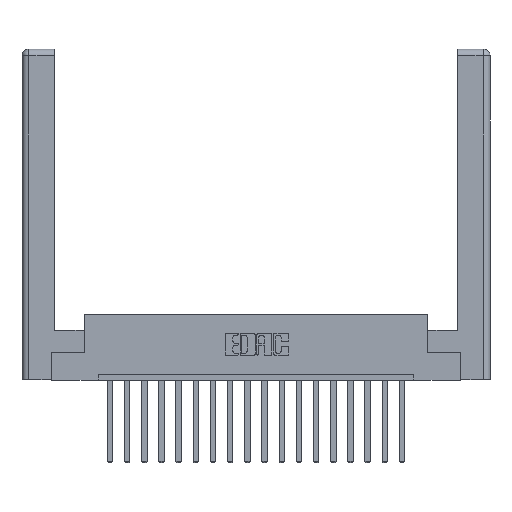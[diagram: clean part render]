
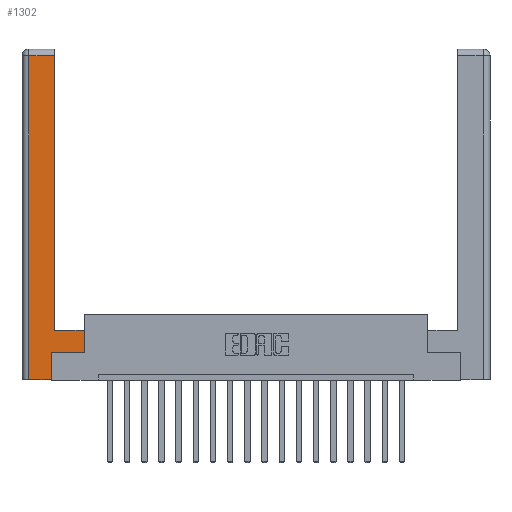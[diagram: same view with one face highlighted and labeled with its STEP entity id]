
A CAD part, top view. The second image highlights one B-rep face of the part: STEP entity #1302.
In plain terms, the highlighted planar face has unit normal (0, 0, 1).
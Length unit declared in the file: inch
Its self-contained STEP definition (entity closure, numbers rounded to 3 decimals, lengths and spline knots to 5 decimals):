
#709 = ORIENTED_EDGE ( 'NONE', *, *, #9413, .T. ) ;
#1058 = VECTOR ( 'NONE', #8706, 39.37008 ) ;
#1302 = ADVANCED_FACE ( 'NONE', ( #15863 ), #8562, .F. ) ;
#1546 = CARTESIAN_POINT ( 'NONE',  ( 0.565, 0.245, 0. ) ) ;
#1646 = VERTEX_POINT ( 'NONE', #6584 ) ;
#2027 = EDGE_CURVE ( 'NONE', #1646, #18087, #2345, .T. ) ;
#2048 = CARTESIAN_POINT ( 'NONE',  ( 0.265, 0., 0. ) ) ;
#2218 = EDGE_CURVE ( 'NONE', #15496, #9915, #7611, .T. ) ;
#2339 = DIRECTION ( 'NONE',  ( 0., 1., 0. ) ) ;
#2345 = LINE ( 'NONE', #8166, #11523 ) ;
#2350 = LINE ( 'NONE', #13489, #13578 ) ;
#2650 = CARTESIAN_POINT ( 'NONE',  ( 0.0615, 2.94, 0. ) ) ;
#2693 = CARTESIAN_POINT ( 'NONE',  ( 0.265, 0., 0. ) ) ;
#2729 = DIRECTION ( 'NONE',  ( -1., 0., 0. ) ) ;
#3001 = DIRECTION ( 'NONE',  ( 1., 0., 0. ) ) ;
#3193 = VECTOR ( 'NONE', #13538, 39.37008 ) ;
#3592 = EDGE_CURVE ( 'NONE', #9915, #18809, #2350, .T. ) ;
#4389 = CARTESIAN_POINT ( 'NONE',  ( 0.0615, 0., 0. ) ) ;
#4455 = ORIENTED_EDGE ( 'NONE', *, *, #3592, .T. ) ;
#4514 = DIRECTION ( 'NONE',  ( 0., 1., 0. ) ) ;
#4628 = VERTEX_POINT ( 'NONE', #2693 ) ;
#4725 = ORIENTED_EDGE ( 'NONE', *, *, #18942, .T. ) ;
#5455 = CARTESIAN_POINT ( 'NONE',  ( 0.0615, 0., 0. ) ) ;
#6584 = CARTESIAN_POINT ( 'NONE',  ( 0.295, 0.45, 0. ) ) ;
#7130 = CARTESIAN_POINT ( 'NONE',  ( 0., 0., 0. ) ) ;
#7320 = LINE ( 'NONE', #2048, #8725 ) ;
#7611 = LINE ( 'NONE', #1546, #9930 ) ;
#8067 = CARTESIAN_POINT ( 'NONE',  ( 0.0615, 2.94, 0. ) ) ;
#8166 = CARTESIAN_POINT ( 'NONE',  ( 0.295, 3., 0. ) ) ;
#8175 = VECTOR ( 'NONE', #17432, 39.37008 ) ;
#8516 = VERTEX_POINT ( 'NONE', #8067 ) ;
#8562 = PLANE ( 'NONE',  #10158 ) ;
#8706 = DIRECTION ( 'NONE',  ( 0., -1., 0. ) ) ;
#8714 = LINE ( 'NONE', #2650, #9632 ) ;
#8725 = VECTOR ( 'NONE', #14958, 39.37008 ) ;
#9068 = CARTESIAN_POINT ( 'NONE',  ( 0.265, 0.245, 0. ) ) ;
#9328 = LINE ( 'NONE', #4389, #1058 ) ;
#9413 = EDGE_CURVE ( 'NONE', #4628, #15496, #12985, .T. ) ;
#9632 = VECTOR ( 'NONE', #14292, 39.37008 ) ;
#9915 = VERTEX_POINT ( 'NONE', #14558 ) ;
#9930 = VECTOR ( 'NONE', #3001, 39.37008 ) ;
#10158 = AXIS2_PLACEMENT_3D ( 'NONE', #7130, #14496, #2729 ) ;
#10539 = CARTESIAN_POINT ( 'NONE',  ( 0.295, 0.45, 0. ) ) ;
#10904 = ORIENTED_EDGE ( 'NONE', *, *, #2218, .T. ) ;
#11028 = ORIENTED_EDGE ( 'NONE', *, *, #12440, .T. ) ;
#11227 = CARTESIAN_POINT ( 'NONE',  ( 0.295, 2.94, 0. ) ) ;
#11523 = VECTOR ( 'NONE', #2339, 39.37008 ) ;
#12440 = EDGE_CURVE ( 'NONE', #18087, #8516, #8714, .T. ) ;
#12825 = LINE ( 'NONE', #10539, #3193 ) ;
#12985 = LINE ( 'NONE', #18950, #8175 ) ;
#13014 = ORIENTED_EDGE ( 'NONE', *, *, #2027, .T. ) ;
#13489 = CARTESIAN_POINT ( 'NONE',  ( 0.565, 0.45, 0. ) ) ;
#13538 = DIRECTION ( 'NONE',  ( -1., 0., 0. ) ) ;
#13578 = VECTOR ( 'NONE', #4514, 39.37008 ) ;
#13657 = VERTEX_POINT ( 'NONE', #5455 ) ;
#13859 = ORIENTED_EDGE ( 'NONE', *, *, #17811, .T. ) ;
#14292 = DIRECTION ( 'NONE',  ( -1., 0., 0. ) ) ;
#14496 = DIRECTION ( 'NONE',  ( 0., 0., -1. ) ) ;
#14558 = CARTESIAN_POINT ( 'NONE',  ( 0.565, 0.245, 0. ) ) ;
#14958 = DIRECTION ( 'NONE',  ( 1., 0., 0. ) ) ;
#14987 = EDGE_CURVE ( 'NONE', #8516, #13657, #9328, .T. ) ;
#15214 = CARTESIAN_POINT ( 'NONE',  ( 0.565, 0.45, 0. ) ) ;
#15496 = VERTEX_POINT ( 'NONE', #9068 ) ;
#15863 = FACE_OUTER_BOUND ( 'NONE', #16887, .T. ) ;
#16887 = EDGE_LOOP ( 'NONE', ( #13014, #11028, #18031, #13859, #709, #10904, #4455, #4725 ) ) ;
#17432 = DIRECTION ( 'NONE',  ( 0., 1., 0. ) ) ;
#17811 = EDGE_CURVE ( 'NONE', #13657, #4628, #7320, .T. ) ;
#18031 = ORIENTED_EDGE ( 'NONE', *, *, #14987, .T. ) ;
#18087 = VERTEX_POINT ( 'NONE', #11227 ) ;
#18809 = VERTEX_POINT ( 'NONE', #15214 ) ;
#18942 = EDGE_CURVE ( 'NONE', #18809, #1646, #12825, .T. ) ;
#18950 = CARTESIAN_POINT ( 'NONE',  ( 0.265, 0.245, 0. ) ) ;
